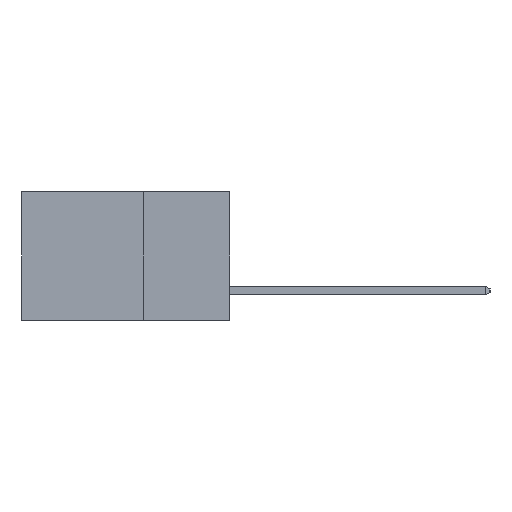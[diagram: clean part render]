
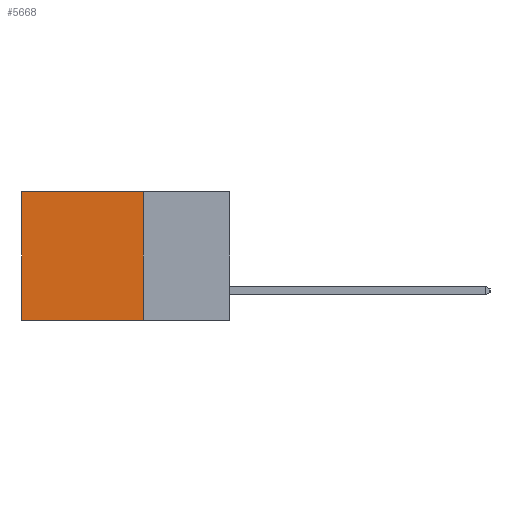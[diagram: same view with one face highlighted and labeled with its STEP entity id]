
A CAD part, left-side view. The second image highlights one B-rep face of the part: STEP entity #5668.
In plain terms, the highlighted planar face has unit normal (-1, 0, 0).
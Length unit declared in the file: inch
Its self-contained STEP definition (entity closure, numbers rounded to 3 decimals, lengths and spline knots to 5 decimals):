
#3074 = CARTESIAN_POINT ( 'NONE',  ( 0.298, 0.25, -0.37 ) ) ;
#3593 = AXIS2_PLACEMENT_3D ( 'NONE', #14801, #13356, #9499 ) ;
#4245 = VECTOR ( 'NONE', #11542, 39.37008 ) ;
#4531 = ORIENTED_EDGE ( 'NONE', *, *, #19527, .T. ) ;
#4905 = EDGE_LOOP ( 'NONE', ( #15334, #17581, #7928, #4531 ) ) ;
#5016 = CARTESIAN_POINT ( 'NONE',  ( 0.298, 0.6, -0.37 ) ) ;
#5023 = PLANE ( 'NONE',  #3593 ) ;
#5090 = VECTOR ( 'NONE', #6500, 39.37008 ) ;
#5668 = ADVANCED_FACE ( 'NONE', ( #6717 ), #5023, .F. ) ;
#5813 = CARTESIAN_POINT ( 'NONE',  ( 0.298, 0.25, -0.37 ) ) ;
#6500 = DIRECTION ( 'NONE',  ( 0., 0., -1. ) ) ;
#6717 = FACE_OUTER_BOUND ( 'NONE', #4905, .T. ) ;
#7120 = LINE ( 'NONE', #7450, #18489 ) ;
#7297 = EDGE_CURVE ( 'NONE', #9226, #7379, #7120, .T. ) ;
#7308 = LINE ( 'NONE', #5813, #14836 ) ;
#7379 = VERTEX_POINT ( 'NONE', #3074 ) ;
#7450 = CARTESIAN_POINT ( 'NONE',  ( 0.298, 0.25, 0. ) ) ;
#7928 = ORIENTED_EDGE ( 'NONE', *, *, #7297, .F. ) ;
#8450 = CARTESIAN_POINT ( 'NONE',  ( 0.298, 0.6, 0. ) ) ;
#8840 = DIRECTION ( 'NONE',  ( 0., 1., 0. ) ) ;
#8902 = CARTESIAN_POINT ( 'NONE',  ( 0.298, 0.25, 0. ) ) ;
#8999 = VERTEX_POINT ( 'NONE', #8450 ) ;
#9226 = VERTEX_POINT ( 'NONE', #8902 ) ;
#9499 = DIRECTION ( 'NONE',  ( 0., 0., -1. ) ) ;
#9508 = CARTESIAN_POINT ( 'NONE',  ( 0.298, 0.6, 0. ) ) ;
#11542 = DIRECTION ( 'NONE',  ( 0., 1., 0. ) ) ;
#12616 = LINE ( 'NONE', #9508, #5090 ) ;
#13356 = DIRECTION ( 'NONE',  ( 1., 0., 0. ) ) ;
#13513 = EDGE_CURVE ( 'NONE', #7379, #16073, #7308, .T. ) ;
#14801 = CARTESIAN_POINT ( 'NONE',  ( 0.298, 0.25, 0. ) ) ;
#14836 = VECTOR ( 'NONE', #8840, 39.37008 ) ;
#15334 = ORIENTED_EDGE ( 'NONE', *, *, #15475, .T. ) ;
#15475 = EDGE_CURVE ( 'NONE', #8999, #16073, #12616, .T. ) ;
#15795 = LINE ( 'NONE', #18881, #4245 ) ;
#16073 = VERTEX_POINT ( 'NONE', #5016 ) ;
#17581 = ORIENTED_EDGE ( 'NONE', *, *, #13513, .F. ) ;
#17870 = DIRECTION ( 'NONE',  ( 0., 0., -1. ) ) ;
#18489 = VECTOR ( 'NONE', #17870, 39.37008 ) ;
#18881 = CARTESIAN_POINT ( 'NONE',  ( 0.298, 0.25, 0. ) ) ;
#19527 = EDGE_CURVE ( 'NONE', #9226, #8999, #15795, .T. ) ;
